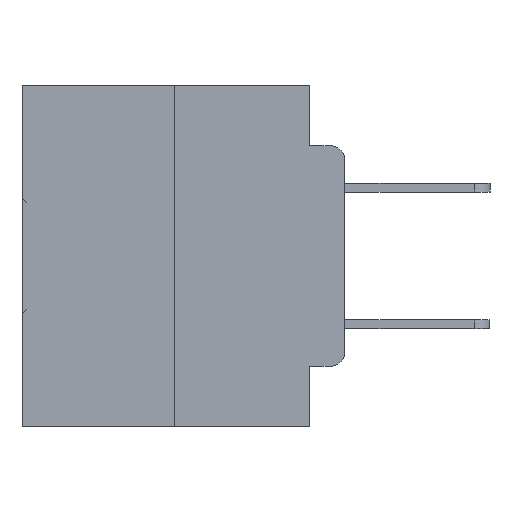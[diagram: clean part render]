
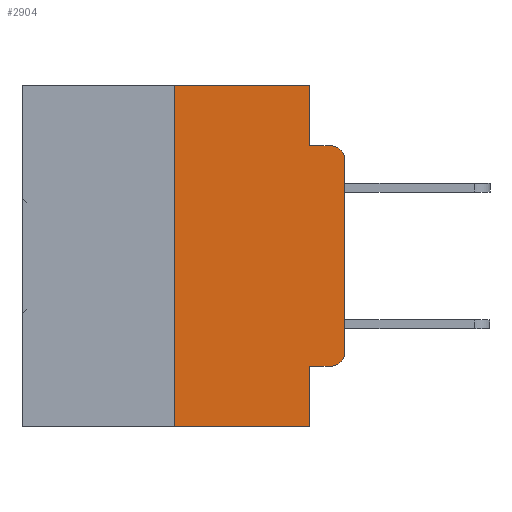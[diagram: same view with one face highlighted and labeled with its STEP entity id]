
A CAD part, left-side view. The second image highlights one B-rep face of the part: STEP entity #2904.
In plain terms, the highlighted planar face has unit normal (-1, 0, 0).
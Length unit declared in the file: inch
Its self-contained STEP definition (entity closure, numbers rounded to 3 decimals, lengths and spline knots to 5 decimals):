
#49 = CARTESIAN_POINT ( 'NONE',  ( 0., 0.473, 0. ) ) ;
#309 = DIRECTION ( 'NONE',  ( 0., 0., -1. ) ) ;
#966 = ORIENTED_EDGE ( 'NONE', *, *, #33546, .T. ) ;
#1821 = ORIENTED_EDGE ( 'NONE', *, *, #17323, .F. ) ;
#2131 = VERTEX_POINT ( 'NONE', #12344 ) ;
#2468 = CARTESIAN_POINT ( 'NONE',  ( 0., 0.051, -0.4115 ) ) ;
#2574 = VECTOR ( 'NONE', #21567, 39.37008 ) ;
#2648 = CARTESIAN_POINT ( 'NONE',  ( 0., 0.051, -0.0885 ) ) ;
#2904 = ADVANCED_FACE ( 'NONE', ( #3429 ), #32330, .F. ) ;
#3014 = ORIENTED_EDGE ( 'NONE', *, *, #31196, .F. ) ;
#3318 = DIRECTION ( 'NONE',  ( 0., 0., 1. ) ) ;
#3429 = FACE_OUTER_BOUND ( 'NONE', #13521, .T. ) ;
#4107 = ORIENTED_EDGE ( 'NONE', *, *, #21432, .T. ) ;
#4292 = ORIENTED_EDGE ( 'NONE', *, *, #4742, .T. ) ;
#4742 = EDGE_CURVE ( 'NONE', #2131, #26391, #32536, .T. ) ;
#4852 = CARTESIAN_POINT ( 'NONE',  ( 0., 0.051, -0.4115 ) ) ;
#4880 = VERTEX_POINT ( 'NONE', #8900 ) ;
#5287 = DIRECTION ( 'NONE',  ( 0., -1., 0. ) ) ;
#6279 = AXIS2_PLACEMENT_3D ( 'NONE', #31651, #16165, #309 ) ;
#7548 = DIRECTION ( 'NONE',  ( 0., -1., 0. ) ) ;
#7606 = DIRECTION ( 'NONE',  ( 0., 0., -1. ) ) ;
#7753 = ORIENTED_EDGE ( 'NONE', *, *, #12049, .F. ) ;
#7921 = DIRECTION ( 'NONE',  ( 0., -1., 0. ) ) ;
#8900 = CARTESIAN_POINT ( 'NONE',  ( 0., 0.02, -0.4115 ) ) ;
#9126 = CARTESIAN_POINT ( 'NONE',  ( 0., 0.473, -0.5 ) ) ;
#9433 = EDGE_CURVE ( 'NONE', #23779, #22381, #33034, .T. ) ;
#9456 = CARTESIAN_POINT ( 'NONE',  ( 0., 0.02, -0.0885 ) ) ;
#9656 = LINE ( 'NONE', #16352, #2574 ) ;
#9797 = VECTOR ( 'NONE', #3318, 39.37008 ) ;
#9989 = EDGE_CURVE ( 'NONE', #31670, #20525, #9656, .T. ) ;
#10456 = VECTOR ( 'NONE', #7606, 39.37008 ) ;
#10648 = CARTESIAN_POINT ( 'NONE',  ( 0., 0., -0.3915 ) ) ;
#11979 = VECTOR ( 'NONE', #7548, 39.37008 ) ;
#12049 = EDGE_CURVE ( 'NONE', #27648, #26391, #31139, .T. ) ;
#12344 = CARTESIAN_POINT ( 'NONE',  ( 0., 0.25, -0.5 ) ) ;
#12838 = CARTESIAN_POINT ( 'NONE',  ( 0., 0.051, 0. ) ) ;
#13144 = CARTESIAN_POINT ( 'NONE',  ( 0., 0.051, 0. ) ) ;
#13432 = CARTESIAN_POINT ( 'NONE',  ( 0., 0.02, -0.3915 ) ) ;
#13521 = EDGE_LOOP ( 'NONE', ( #27821, #20057, #18905, #3014, #33304, #1821, #4292, #7753, #966, #4107 ) ) ;
#14219 = VECTOR ( 'NONE', #19075, 39.37008 ) ;
#14323 = CIRCLE ( 'NONE', #21742, 0.02 ) ;
#14752 = CARTESIAN_POINT ( 'NONE',  ( 0., 0.051, 0. ) ) ;
#14776 = CARTESIAN_POINT ( 'NONE',  ( 0., 0.25, 0. ) ) ;
#15804 = DIRECTION ( 'NONE',  ( 0., 0., -1. ) ) ;
#16075 = DIRECTION ( 'NONE',  ( 0., 0., -1. ) ) ;
#16165 = DIRECTION ( 'NONE',  ( -1., 0., 0. ) ) ;
#16352 = CARTESIAN_POINT ( 'NONE',  ( 0., 0.473, 0. ) ) ;
#17154 = VECTOR ( 'NONE', #7921, 39.37008 ) ;
#17323 = EDGE_CURVE ( 'NONE', #2131, #31670, #32464, .T. ) ;
#17536 = DIRECTION ( 'NONE',  ( 1., 0., 0. ) ) ;
#18201 = LINE ( 'NONE', #2648, #25147 ) ;
#18384 = EDGE_CURVE ( 'NONE', #25600, #22381, #18201, .T. ) ;
#18905 = ORIENTED_EDGE ( 'NONE', *, *, #18384, .F. ) ;
#19051 = VERTEX_POINT ( 'NONE', #10648 ) ;
#19075 = DIRECTION ( 'NONE',  ( 0., 0., 1. ) ) ;
#20057 = ORIENTED_EDGE ( 'NONE', *, *, #9433, .T. ) ;
#20525 = VERTEX_POINT ( 'NONE', #14752 ) ;
#21432 = EDGE_CURVE ( 'NONE', #4880, #19051, #14323, .T. ) ;
#21567 = DIRECTION ( 'NONE',  ( 0., -1., 0. ) ) ;
#21742 = AXIS2_PLACEMENT_3D ( 'NONE', #13432, #31564, #16075 ) ;
#22381 = VERTEX_POINT ( 'NONE', #9456 ) ;
#23466 = EDGE_CURVE ( 'NONE', #19051, #23779, #31364, .T. ) ;
#23779 = VERTEX_POINT ( 'NONE', #33234 ) ;
#25147 = VECTOR ( 'NONE', #5287, 39.37008 ) ;
#25168 = LINE ( 'NONE', #12838, #10456 ) ;
#25600 = VERTEX_POINT ( 'NONE', #25720 ) ;
#25720 = CARTESIAN_POINT ( 'NONE',  ( 0., 0.051, -0.0885 ) ) ;
#26391 = VERTEX_POINT ( 'NONE', #28570 ) ;
#26991 = CARTESIAN_POINT ( 'NONE',  ( 0., 0., 0. ) ) ;
#27648 = VERTEX_POINT ( 'NONE', #2468 ) ;
#27821 = ORIENTED_EDGE ( 'NONE', *, *, #23466, .T. ) ;
#27872 = AXIS2_PLACEMENT_3D ( 'NONE', #49, #17536, #33246 ) ;
#28570 = CARTESIAN_POINT ( 'NONE',  ( 0., 0.051, -0.5 ) ) ;
#30344 = VECTOR ( 'NONE', #15804, 39.37008 ) ;
#31139 = LINE ( 'NONE', #13144, #30344 ) ;
#31196 = EDGE_CURVE ( 'NONE', #20525, #25600, #25168, .T. ) ;
#31364 = LINE ( 'NONE', #26991, #9797 ) ;
#31564 = DIRECTION ( 'NONE',  ( -1., 0., 0. ) ) ;
#31651 = CARTESIAN_POINT ( 'NONE',  ( 0., 0.02, -0.1085 ) ) ;
#31670 = VERTEX_POINT ( 'NONE', #14776 ) ;
#31996 = CARTESIAN_POINT ( 'NONE',  ( 0., 0.25, 0. ) ) ;
#32330 = PLANE ( 'NONE',  #27872 ) ;
#32464 = LINE ( 'NONE', #31996, #14219 ) ;
#32536 = LINE ( 'NONE', #9126, #17154 ) ;
#32687 = LINE ( 'NONE', #4852, #11979 ) ;
#33034 = CIRCLE ( 'NONE', #6279, 0.02 ) ;
#33234 = CARTESIAN_POINT ( 'NONE',  ( 0., 0., -0.1085 ) ) ;
#33246 = DIRECTION ( 'NONE',  ( 0., 0., -1. ) ) ;
#33304 = ORIENTED_EDGE ( 'NONE', *, *, #9989, .F. ) ;
#33546 = EDGE_CURVE ( 'NONE', #27648, #4880, #32687, .T. ) ;
